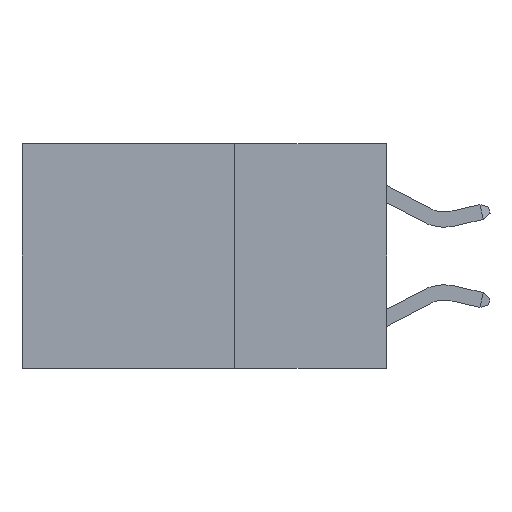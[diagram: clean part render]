
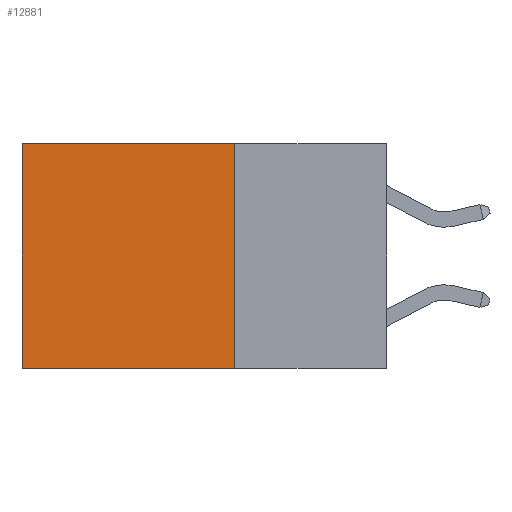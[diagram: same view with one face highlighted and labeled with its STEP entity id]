
A CAD part, left-side view. The second image highlights one B-rep face of the part: STEP entity #12881.
In plain terms, the highlighted planar face has unit normal (-1, 0, 0).
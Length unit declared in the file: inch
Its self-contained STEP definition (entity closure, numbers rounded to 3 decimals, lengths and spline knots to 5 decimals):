
#52 = DIRECTION ( 'NONE',  ( 0., 0., -1. ) ) ;
#228 = CARTESIAN_POINT ( 'NONE',  ( 0.2625, 0.25, -0.37 ) ) ;
#2303 = LINE ( 'NONE', #12525, #12859 ) ;
#2357 = CARTESIAN_POINT ( 'NONE',  ( 0.2625, 0.25, 0. ) ) ;
#2667 = EDGE_CURVE ( 'NONE', #3075, #28941, #24383, .T. ) ;
#2878 = AXIS2_PLACEMENT_3D ( 'NONE', #4583, #22771, #9203 ) ;
#3075 = VERTEX_POINT ( 'NONE', #2357 ) ;
#3765 = CARTESIAN_POINT ( 'NONE',  ( 0.2625, 0.25, 0. ) ) ;
#4583 = CARTESIAN_POINT ( 'NONE',  ( 0.2625, 0.25, 0. ) ) ;
#6869 = VERTEX_POINT ( 'NONE', #7597 ) ;
#6897 = CARTESIAN_POINT ( 'NONE',  ( 0.2625, 0.6, 0. ) ) ;
#7597 = CARTESIAN_POINT ( 'NONE',  ( 0.2625, 0.25, -0.37 ) ) ;
#9203 = DIRECTION ( 'NONE',  ( 0., 0., -1. ) ) ;
#9452 = VECTOR ( 'NONE', #52, 39.37008 ) ;
#10163 = FACE_OUTER_BOUND ( 'NONE', #12459, .T. ) ;
#10657 = ORIENTED_EDGE ( 'NONE', *, *, #28412, .F. ) ;
#12459 = EDGE_LOOP ( 'NONE', ( #20329, #10657, #14249, #13456 ) ) ;
#12525 = CARTESIAN_POINT ( 'NONE',  ( 0.2625, 0.25, 0. ) ) ;
#12799 = DIRECTION ( 'NONE',  ( 0., 1., 0. ) ) ;
#12859 = VECTOR ( 'NONE', #17029, 39.37008 ) ;
#12881 = ADVANCED_FACE ( 'NONE', ( #10163 ), #15576, .F. ) ;
#13456 = ORIENTED_EDGE ( 'NONE', *, *, #2667, .T. ) ;
#14154 = CARTESIAN_POINT ( 'NONE',  ( 0.2625, 0.6, 0. ) ) ;
#14249 = ORIENTED_EDGE ( 'NONE', *, *, #18882, .F. ) ;
#15576 = PLANE ( 'NONE',  #2878 ) ;
#16070 = DIRECTION ( 'NONE',  ( 0., 1., 0. ) ) ;
#17029 = DIRECTION ( 'NONE',  ( 0., 0., -1. ) ) ;
#18401 = VECTOR ( 'NONE', #12799, 39.37008 ) ;
#18882 = EDGE_CURVE ( 'NONE', #3075, #6869, #2303, .T. ) ;
#20329 = ORIENTED_EDGE ( 'NONE', *, *, #27745, .T. ) ;
#20373 = CARTESIAN_POINT ( 'NONE',  ( 0.2625, 0.6, -0.37 ) ) ;
#20441 = LINE ( 'NONE', #228, #24681 ) ;
#21151 = VERTEX_POINT ( 'NONE', #20373 ) ;
#22771 = DIRECTION ( 'NONE',  ( 1., 0., 0. ) ) ;
#24383 = LINE ( 'NONE', #3765, #18401 ) ;
#24681 = VECTOR ( 'NONE', #16070, 39.37008 ) ;
#27745 = EDGE_CURVE ( 'NONE', #28941, #21151, #28894, .T. ) ;
#28412 = EDGE_CURVE ( 'NONE', #6869, #21151, #20441, .T. ) ;
#28894 = LINE ( 'NONE', #6897, #9452 ) ;
#28941 = VERTEX_POINT ( 'NONE', #14154 ) ;
